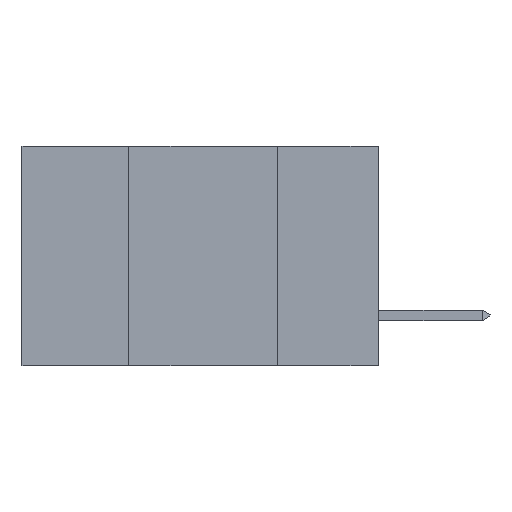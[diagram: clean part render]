
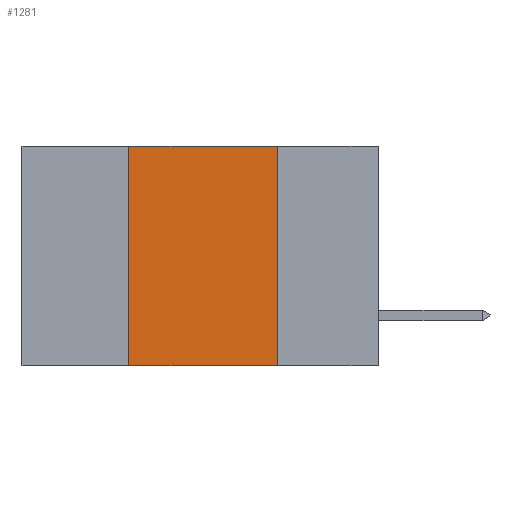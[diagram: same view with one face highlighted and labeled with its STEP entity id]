
A CAD part, left-side view. The second image highlights one B-rep face of the part: STEP entity #1281.
In plain terms, the highlighted planar face has unit normal (-1, 0, 0).
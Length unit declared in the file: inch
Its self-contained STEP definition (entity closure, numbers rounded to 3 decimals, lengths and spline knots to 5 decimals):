
#77 = ORIENTED_EDGE ( 'NONE', *, *, #10656, .T. ) ;
#684 = CARTESIAN_POINT ( 'NONE',  ( 0., 0.6, -0.37 ) ) ;
#731 = DIRECTION ( 'NONE',  ( 0., -1., 0. ) ) ;
#766 = CARTESIAN_POINT ( 'NONE',  ( 0., 0.42, 0. ) ) ;
#814 = DIRECTION ( 'NONE',  ( 0., 0., 1. ) ) ;
#1068 = DIRECTION ( 'NONE',  ( 0., -1., 0. ) ) ;
#1281 = ADVANCED_FACE ( 'NONE', ( #12592 ), #4485, .F. ) ;
#1544 = LINE ( 'NONE', #11477, #11493 ) ;
#1620 = VECTOR ( 'NONE', #814, 39.37008 ) ;
#1703 = ORIENTED_EDGE ( 'NONE', *, *, #14290, .F. ) ;
#2447 = CARTESIAN_POINT ( 'NONE',  ( 0., 0.42, -0.37 ) ) ;
#3523 = VECTOR ( 'NONE', #1068, 39.37008 ) ;
#4485 = PLANE ( 'NONE',  #10590 ) ;
#4571 = CARTESIAN_POINT ( 'NONE',  ( 0., 0.6, 0. ) ) ;
#4912 = EDGE_CURVE ( 'NONE', #6801, #7421, #7471, .T. ) ;
#5447 = VERTEX_POINT ( 'NONE', #12692 ) ;
#6085 = EDGE_CURVE ( 'NONE', #9894, #6801, #12801, .T. ) ;
#6658 = CARTESIAN_POINT ( 'NONE',  ( 0., 0.42, 0. ) ) ;
#6801 = VERTEX_POINT ( 'NONE', #6658 ) ;
#7110 = EDGE_LOOP ( 'NONE', ( #1703, #7262, #14207, #77 ) ) ;
#7262 = ORIENTED_EDGE ( 'NONE', *, *, #4912, .F. ) ;
#7421 = VERTEX_POINT ( 'NONE', #13918 ) ;
#7471 = LINE ( 'NONE', #11587, #3523 ) ;
#8429 = LINE ( 'NONE', #684, #9968 ) ;
#9894 = VERTEX_POINT ( 'NONE', #2447 ) ;
#9968 = VECTOR ( 'NONE', #731, 39.37008 ) ;
#10001 = DIRECTION ( 'NONE',  ( 1., 0., 0. ) ) ;
#10590 = AXIS2_PLACEMENT_3D ( 'NONE', #4571, #10001, #12236 ) ;
#10656 = EDGE_CURVE ( 'NONE', #9894, #5447, #8429, .T. ) ;
#11477 = CARTESIAN_POINT ( 'NONE',  ( 0., 0.17, 0. ) ) ;
#11493 = VECTOR ( 'NONE', #12558, 39.37008 ) ;
#11587 = CARTESIAN_POINT ( 'NONE',  ( 0., 0.6, 0. ) ) ;
#12236 = DIRECTION ( 'NONE',  ( 0., 0., -1. ) ) ;
#12558 = DIRECTION ( 'NONE',  ( 0., 0., -1. ) ) ;
#12592 = FACE_OUTER_BOUND ( 'NONE', #7110, .T. ) ;
#12692 = CARTESIAN_POINT ( 'NONE',  ( 0., 0.17, -0.37 ) ) ;
#12801 = LINE ( 'NONE', #766, #1620 ) ;
#13918 = CARTESIAN_POINT ( 'NONE',  ( 0., 0.17, 0. ) ) ;
#14207 = ORIENTED_EDGE ( 'NONE', *, *, #6085, .F. ) ;
#14290 = EDGE_CURVE ( 'NONE', #7421, #5447, #1544, .T. ) ;
